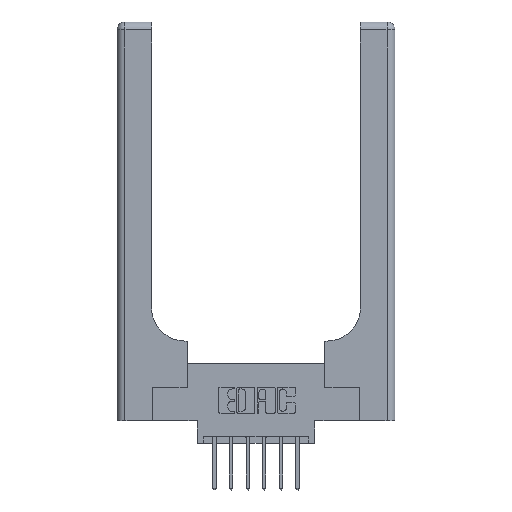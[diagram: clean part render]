
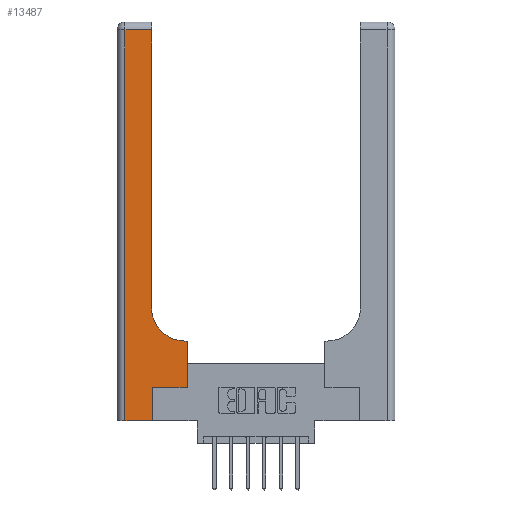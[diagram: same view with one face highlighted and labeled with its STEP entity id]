
A CAD part, top view. The second image highlights one B-rep face of the part: STEP entity #13487.
In plain terms, the highlighted planar face has unit normal (0, 0, 1).
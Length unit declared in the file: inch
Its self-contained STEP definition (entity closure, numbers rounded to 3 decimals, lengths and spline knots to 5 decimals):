
#66 = LINE ( 'NONE', #8356, #4810 ) ;
#220 = CARTESIAN_POINT ( 'NONE',  ( 0.528, 0.25, 0.37 ) ) ;
#791 = DIRECTION ( 'NONE',  ( 0., 1., 0. ) ) ;
#849 = DIRECTION ( 'NONE',  ( -1., 0., 0. ) ) ;
#890 = LINE ( 'NONE', #9781, #8892 ) ;
#1084 = VECTOR ( 'NONE', #6731, 39.37008 ) ;
#1422 = DIRECTION ( 'NONE',  ( -1., 0., 0. ) ) ;
#1528 = LINE ( 'NONE', #12655, #12299 ) ;
#2056 = VECTOR ( 'NONE', #12837, 39.37008 ) ;
#2294 = DIRECTION ( 'NONE',  ( 1., 0., 0. ) ) ;
#2370 = EDGE_CURVE ( 'NONE', #2701, #3459, #4471, .T. ) ;
#2701 = VERTEX_POINT ( 'NONE', #9718 ) ;
#2875 = VERTEX_POINT ( 'NONE', #220 ) ;
#3394 = CARTESIAN_POINT ( 'NONE',  ( 0.265, 0.25, 0.37 ) ) ;
#3459 = VERTEX_POINT ( 'NONE', #7188 ) ;
#3695 = ORIENTED_EDGE ( 'NONE', *, *, #4121, .T. ) ;
#4121 = EDGE_CURVE ( 'NONE', #8109, #12062, #4947, .T. ) ;
#4471 = LINE ( 'NONE', #12576, #7026 ) ;
#4810 = VECTOR ( 'NONE', #791, 39.37008 ) ;
#4947 = LINE ( 'NONE', #5208, #2056 ) ;
#5084 = AXIS2_PLACEMENT_3D ( 'NONE', #13370, #7950, #1422 ) ;
#5169 = CARTESIAN_POINT ( 'NONE',  ( 0.51, 0.85, 0.37 ) ) ;
#5174 = LINE ( 'NONE', #13941, #13512 ) ;
#5208 = CARTESIAN_POINT ( 'NONE',  ( 0., 0., 0.37 ) ) ;
#5752 = PLANE ( 'NONE',  #5084 ) ;
#6032 = DIRECTION ( 'NONE',  ( -1., 0., 0. ) ) ;
#6108 = ORIENTED_EDGE ( 'NONE', *, *, #2370, .T. ) ;
#6272 = DIRECTION ( 'NONE',  ( 1., 0., 0. ) ) ;
#6726 = CARTESIAN_POINT ( 'NONE',  ( 0.51, 0.6, 0.37 ) ) ;
#6731 = DIRECTION ( 'NONE',  ( 0., -1., 0. ) ) ;
#7026 = VECTOR ( 'NONE', #6032, 39.37008 ) ;
#7188 = CARTESIAN_POINT ( 'NONE',  ( 0.06, 2.94, 0.37 ) ) ;
#7464 = CARTESIAN_POINT ( 'NONE',  ( 0.265, 0.25, 0.37 ) ) ;
#7472 = ORIENTED_EDGE ( 'NONE', *, *, #11507, .T. ) ;
#7499 = ORIENTED_EDGE ( 'NONE', *, *, #11445, .T. ) ;
#7950 = DIRECTION ( 'NONE',  ( 0., 0., -1. ) ) ;
#8029 = CARTESIAN_POINT ( 'NONE',  ( 0.26, 0.85, 0.37 ) ) ;
#8109 = VERTEX_POINT ( 'NONE', #9530 ) ;
#8356 = CARTESIAN_POINT ( 'NONE',  ( 0.265, 0., 0.37 ) ) ;
#8419 = CIRCLE ( 'NONE', #8750, 0.25 ) ;
#8487 = VERTEX_POINT ( 'NONE', #7464 ) ;
#8550 = LINE ( 'NONE', #3394, #11790 ) ;
#8689 = VERTEX_POINT ( 'NONE', #12671 ) ;
#8706 = FACE_OUTER_BOUND ( 'NONE', #12091, .T. ) ;
#8750 = AXIS2_PLACEMENT_3D ( 'NONE', #5169, #12796, #6272 ) ;
#8865 = ORIENTED_EDGE ( 'NONE', *, *, #9354, .T. ) ;
#8892 = VECTOR ( 'NONE', #9828, 39.37008 ) ;
#9018 = ORIENTED_EDGE ( 'NONE', *, *, #9895, .T. ) ;
#9354 = EDGE_CURVE ( 'NONE', #11582, #10912, #8419, .T. ) ;
#9408 = EDGE_CURVE ( 'NONE', #8689, #11582, #5174, .T. ) ;
#9530 = CARTESIAN_POINT ( 'NONE',  ( 0.06, 0., 0.37 ) ) ;
#9718 = CARTESIAN_POINT ( 'NONE',  ( 0.26, 2.94, 0.37 ) ) ;
#9781 = CARTESIAN_POINT ( 'NONE',  ( 0.528, 0.25, 0.37 ) ) ;
#9828 = DIRECTION ( 'NONE',  ( 0., 1., 0. ) ) ;
#9851 = ORIENTED_EDGE ( 'NONE', *, *, #10254, .T. ) ;
#9895 = EDGE_CURVE ( 'NONE', #12062, #8487, #66, .T. ) ;
#10015 = CARTESIAN_POINT ( 'NONE',  ( 0.06, 3., 0.37 ) ) ;
#10254 = EDGE_CURVE ( 'NONE', #3459, #8109, #12313, .T. ) ;
#10328 = ORIENTED_EDGE ( 'NONE', *, *, #12402, .T. ) ;
#10912 = VERTEX_POINT ( 'NONE', #8029 ) ;
#11264 = ORIENTED_EDGE ( 'NONE', *, *, #9408, .T. ) ;
#11445 = EDGE_CURVE ( 'NONE', #2875, #8689, #890, .T. ) ;
#11507 = EDGE_CURVE ( 'NONE', #8487, #2875, #8550, .T. ) ;
#11582 = VERTEX_POINT ( 'NONE', #6726 ) ;
#11790 = VECTOR ( 'NONE', #2294, 39.37008 ) ;
#12062 = VERTEX_POINT ( 'NONE', #14099 ) ;
#12091 = EDGE_LOOP ( 'NONE', ( #10328, #6108, #9851, #3695, #9018, #7472, #7499, #11264, #8865 ) ) ;
#12299 = VECTOR ( 'NONE', #13795, 39.37008 ) ;
#12313 = LINE ( 'NONE', #10015, #1084 ) ;
#12402 = EDGE_CURVE ( 'NONE', #10912, #2701, #1528, .T. ) ;
#12576 = CARTESIAN_POINT ( 'NONE',  ( 0., 2.94, 0.37 ) ) ;
#12655 = CARTESIAN_POINT ( 'NONE',  ( 0.26, 3., 0.37 ) ) ;
#12671 = CARTESIAN_POINT ( 'NONE',  ( 0.528, 0.6, 0.37 ) ) ;
#12796 = DIRECTION ( 'NONE',  ( 0., 0., -1. ) ) ;
#12837 = DIRECTION ( 'NONE',  ( 1., 0., 0. ) ) ;
#13370 = CARTESIAN_POINT ( 'NONE',  ( 0., 3., 0.37 ) ) ;
#13487 = ADVANCED_FACE ( 'NONE', ( #8706 ), #5752, .F. ) ;
#13512 = VECTOR ( 'NONE', #849, 39.37008 ) ;
#13795 = DIRECTION ( 'NONE',  ( 0., 1., 0. ) ) ;
#13941 = CARTESIAN_POINT ( 'NONE',  ( 0.26, 0.6, 0.37 ) ) ;
#14099 = CARTESIAN_POINT ( 'NONE',  ( 0.265, 0., 0.37 ) ) ;
